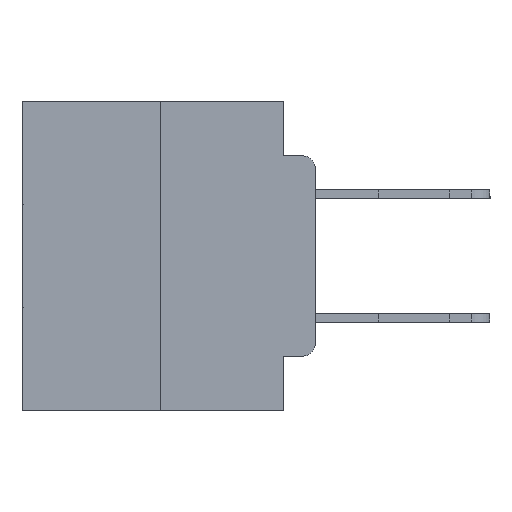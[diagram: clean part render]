
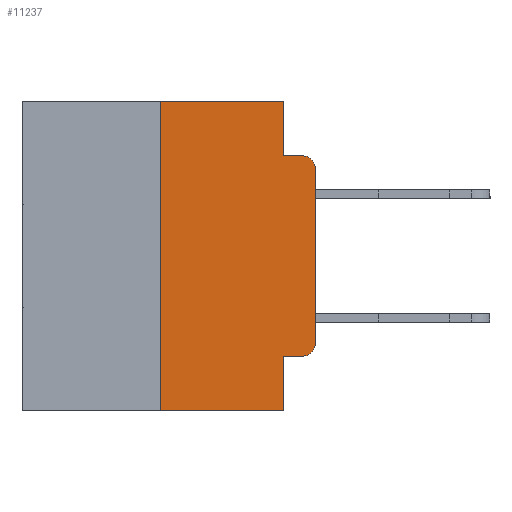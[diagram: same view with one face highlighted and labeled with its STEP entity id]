
A CAD part, left-side view. The second image highlights one B-rep face of the part: STEP entity #11237.
In plain terms, the highlighted planar face has unit normal (-1, 0, 0).
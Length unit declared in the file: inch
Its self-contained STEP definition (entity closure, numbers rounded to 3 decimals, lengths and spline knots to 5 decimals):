
#29 = VERTEX_POINT ( 'NONE', #20822 ) ;
#191 = DIRECTION ( 'NONE',  ( 0., 0., -1. ) ) ;
#838 = CARTESIAN_POINT ( 'NONE',  ( 0., 0.02, -0.3915 ) ) ;
#1211 = VERTEX_POINT ( 'NONE', #21556 ) ;
#1692 = VECTOR ( 'NONE', #3654, 39.37008 ) ;
#1814 = CARTESIAN_POINT ( 'NONE',  ( 0., 0.25, 0. ) ) ;
#2023 = DIRECTION ( 'NONE',  ( 0., 0., -1. ) ) ;
#2262 = ORIENTED_EDGE ( 'NONE', *, *, #4743, .F. ) ;
#2617 = EDGE_LOOP ( 'NONE', ( #22377, #7267, #18206, #12097, #17558, #2262, #24943, #15652, #25588, #4964 ) ) ;
#3040 = DIRECTION ( 'NONE',  ( 0., 0., -1. ) ) ;
#3139 = CARTESIAN_POINT ( 'NONE',  ( 0., 0.02, -0.0885 ) ) ;
#3290 = FACE_OUTER_BOUND ( 'NONE', #2617, .T. ) ;
#3564 = CARTESIAN_POINT ( 'NONE',  ( 0., 0.051, -0.0885 ) ) ;
#3654 = DIRECTION ( 'NONE',  ( 0., -1., 0. ) ) ;
#3742 = LINE ( 'NONE', #3564, #1692 ) ;
#3804 = VERTEX_POINT ( 'NONE', #16376 ) ;
#4099 = EDGE_CURVE ( 'NONE', #5774, #1211, #11962, .T. ) ;
#4131 = CARTESIAN_POINT ( 'NONE',  ( 0., 0.051, 0. ) ) ;
#4717 = CARTESIAN_POINT ( 'NONE',  ( 0., 0., -0.3915 ) ) ;
#4725 = AXIS2_PLACEMENT_3D ( 'NONE', #7377, #21754, #9443 ) ;
#4743 = EDGE_CURVE ( 'NONE', #26545, #29, #14196, .T. ) ;
#4964 = ORIENTED_EDGE ( 'NONE', *, *, #18312, .T. ) ;
#5001 = CARTESIAN_POINT ( 'NONE',  ( 0., 0.051, -0.4115 ) ) ;
#5528 = EDGE_CURVE ( 'NONE', #11960, #15122, #21506, .T. ) ;
#5774 = VERTEX_POINT ( 'NONE', #12650 ) ;
#5783 = LINE ( 'NONE', #4131, #16094 ) ;
#6428 = EDGE_CURVE ( 'NONE', #15030, #3804, #22110, .T. ) ;
#6495 = VECTOR ( 'NONE', #10823, 39.37008 ) ;
#6810 = AXIS2_PLACEMENT_3D ( 'NONE', #16851, #12818, #191 ) ;
#7267 = ORIENTED_EDGE ( 'NONE', *, *, #24319, .T. ) ;
#7377 = CARTESIAN_POINT ( 'NONE',  ( 0., 0.02, -0.1085 ) ) ;
#7623 = CIRCLE ( 'NONE', #4725, 0.02 ) ;
#8338 = CARTESIAN_POINT ( 'NONE',  ( 0., 0.051, 0. ) ) ;
#8616 = DIRECTION ( 'NONE',  ( 0., -1., 0. ) ) ;
#9180 = DIRECTION ( 'NONE',  ( 0., 0., 1. ) ) ;
#9443 = DIRECTION ( 'NONE',  ( 0., 0., -1. ) ) ;
#10823 = DIRECTION ( 'NONE',  ( 0., -1., 0. ) ) ;
#10883 = VECTOR ( 'NONE', #8616, 39.37008 ) ;
#11237 = ADVANCED_FACE ( 'NONE', ( #3290 ), #25101, .F. ) ;
#11259 = LINE ( 'NONE', #26854, #17366 ) ;
#11473 = VERTEX_POINT ( 'NONE', #3139 ) ;
#11960 = VERTEX_POINT ( 'NONE', #4717 ) ;
#11962 = LINE ( 'NONE', #5001, #6495 ) ;
#12019 = VERTEX_POINT ( 'NONE', #13224 ) ;
#12097 = ORIENTED_EDGE ( 'NONE', *, *, #6428, .F. ) ;
#12650 = CARTESIAN_POINT ( 'NONE',  ( 0., 0.051, -0.4115 ) ) ;
#12818 = DIRECTION ( 'NONE',  ( 1., 0., 0. ) ) ;
#13224 = CARTESIAN_POINT ( 'NONE',  ( 0., 0.051, -0.5 ) ) ;
#13284 = EDGE_CURVE ( 'NONE', #26545, #12019, #11259, .T. ) ;
#13302 = EDGE_CURVE ( 'NONE', #5774, #12019, #5783, .T. ) ;
#14196 = LINE ( 'NONE', #1814, #23792 ) ;
#14506 = EDGE_CURVE ( 'NONE', #29, #15030, #25988, .T. ) ;
#14552 = DIRECTION ( 'NONE',  ( 0., -1., 0. ) ) ;
#15030 = VERTEX_POINT ( 'NONE', #8338 ) ;
#15122 = VERTEX_POINT ( 'NONE', #20897 ) ;
#15484 = DIRECTION ( 'NONE',  ( -1., 0., 0. ) ) ;
#15652 = ORIENTED_EDGE ( 'NONE', *, *, #13302, .F. ) ;
#16063 = VECTOR ( 'NONE', #9180, 39.37008 ) ;
#16094 = VECTOR ( 'NONE', #2023, 39.37008 ) ;
#16376 = CARTESIAN_POINT ( 'NONE',  ( 0., 0.051, -0.0885 ) ) ;
#16851 = CARTESIAN_POINT ( 'NONE',  ( 0., 0.473, 0. ) ) ;
#17366 = VECTOR ( 'NONE', #14552, 39.37008 ) ;
#17368 = DIRECTION ( 'NONE',  ( 0., 0., 1. ) ) ;
#17395 = CIRCLE ( 'NONE', #17935, 0.02 ) ;
#17517 = CARTESIAN_POINT ( 'NONE',  ( 0., 0.25, -0.5 ) ) ;
#17558 = ORIENTED_EDGE ( 'NONE', *, *, #14506, .F. ) ;
#17935 = AXIS2_PLACEMENT_3D ( 'NONE', #838, #15484, #3040 ) ;
#18206 = ORIENTED_EDGE ( 'NONE', *, *, #26751, .F. ) ;
#18312 = EDGE_CURVE ( 'NONE', #1211, #11960, #17395, .T. ) ;
#20822 = CARTESIAN_POINT ( 'NONE',  ( 0., 0.25, 0. ) ) ;
#20897 = CARTESIAN_POINT ( 'NONE',  ( 0., 0., -0.1085 ) ) ;
#21506 = LINE ( 'NONE', #24560, #16063 ) ;
#21556 = CARTESIAN_POINT ( 'NONE',  ( 0., 0.02, -0.4115 ) ) ;
#21754 = DIRECTION ( 'NONE',  ( -1., 0., 0. ) ) ;
#22110 = LINE ( 'NONE', #26863, #26949 ) ;
#22377 = ORIENTED_EDGE ( 'NONE', *, *, #5528, .T. ) ;
#23002 = CARTESIAN_POINT ( 'NONE',  ( 0., 0.473, 0. ) ) ;
#23792 = VECTOR ( 'NONE', #17368, 39.37008 ) ;
#24319 = EDGE_CURVE ( 'NONE', #15122, #11473, #7623, .T. ) ;
#24384 = DIRECTION ( 'NONE',  ( 0., 0., -1. ) ) ;
#24560 = CARTESIAN_POINT ( 'NONE',  ( 0., 0., 0. ) ) ;
#24943 = ORIENTED_EDGE ( 'NONE', *, *, #13284, .T. ) ;
#25101 = PLANE ( 'NONE',  #6810 ) ;
#25588 = ORIENTED_EDGE ( 'NONE', *, *, #4099, .T. ) ;
#25988 = LINE ( 'NONE', #23002, #10883 ) ;
#26545 = VERTEX_POINT ( 'NONE', #17517 ) ;
#26751 = EDGE_CURVE ( 'NONE', #3804, #11473, #3742, .T. ) ;
#26854 = CARTESIAN_POINT ( 'NONE',  ( 0., 0.473, -0.5 ) ) ;
#26863 = CARTESIAN_POINT ( 'NONE',  ( 0., 0.051, 0. ) ) ;
#26949 = VECTOR ( 'NONE', #24384, 39.37008 ) ;
